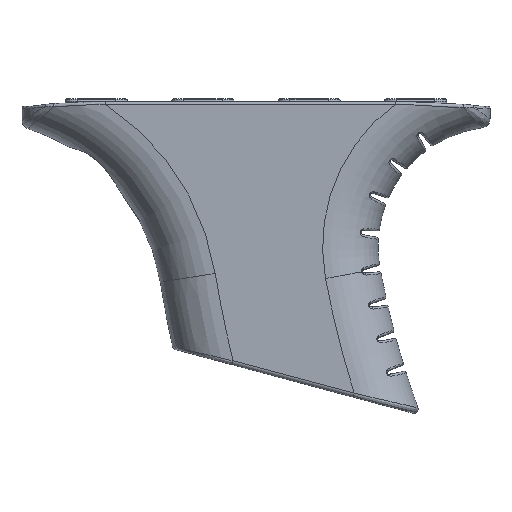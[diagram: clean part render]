
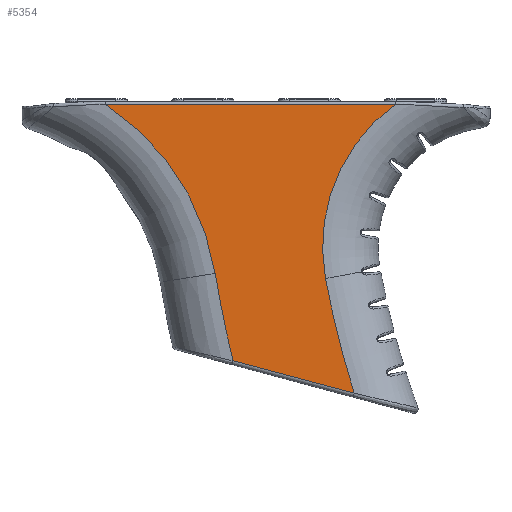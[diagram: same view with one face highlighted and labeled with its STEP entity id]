
A CAD part, left-side view. The second image highlights one B-rep face of the part: STEP entity #5354.
In plain terms, the highlighted planar face has unit normal (-1, 0, 0).
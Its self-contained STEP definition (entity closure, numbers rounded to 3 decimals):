
#47=PLANE('',#5767);
#331=LINE('',#21706,#554);
#336=LINE('',#21870,#559);
#554=VECTOR('',#6568,10.);
#559=VECTOR('',#6621,11.);
#841=FACE_OUTER_BOUND('',#1180,.T.);
#1180=EDGE_LOOP('',(#4352,#4353,#4354,#4355,#4356,#4357));
#1677=CIRCLE('',#5548,33.);
#1707=CIRCLE('',#5583,177.731);
#1833=CIRCLE('',#5761,198.);
#1838=CIRCLE('',#5768,46.75);
#2016=VERTEX_POINT('',#8795);
#2017=VERTEX_POINT('',#8801);
#2103=VERTEX_POINT('',#15218);
#2363=VERTEX_POINT('',#21693);
#2371=VERTEX_POINT('',#21860);
#2373=VERTEX_POINT('',#21869);
#2556=EDGE_CURVE('',#2017,#2016,#1677,.T.);
#2681=EDGE_CURVE('',#2103,#2017,#1707,.T.);
#3042=EDGE_CURVE('',#2103,#2363,#331,.T.);
#3058=EDGE_CURVE('',#2371,#2363,#1833,.T.);
#3063=EDGE_CURVE('',#2373,#2016,#336,.T.);
#3064=EDGE_CURVE('',#2371,#2373,#1838,.T.);
#4352=ORIENTED_EDGE('',*,*,#3042,.F.);
#4353=ORIENTED_EDGE('',*,*,#2681,.T.);
#4354=ORIENTED_EDGE('',*,*,#2556,.T.);
#4355=ORIENTED_EDGE('',*,*,#3063,.F.);
#4356=ORIENTED_EDGE('',*,*,#3064,.F.);
#4357=ORIENTED_EDGE('',*,*,#3058,.T.);
#5354=ADVANCED_FACE('',(#841),#47,.T.);
#5548=AXIS2_PLACEMENT_3D('',#8802,#6082,#6083);
#5583=AXIS2_PLACEMENT_3D('',#15219,#6155,#6156);
#5761=AXIS2_PLACEMENT_3D('',#21861,#6607,#6608);
#5767=AXIS2_PLACEMENT_3D('',#21868,#6619,#6620);
#5768=AXIS2_PLACEMENT_3D('',#21871,#6622,#6623);
#6082=DIRECTION('center_axis',(1.,0.,0.));
#6083=DIRECTION('ref_axis',(0.,0.915,0.402));
#6155=DIRECTION('center_axis',(1.,0.,0.));
#6156=DIRECTION('ref_axis',(0.,0.957,-0.289));
#6568=DIRECTION('',(0.,0.966,0.259));
#6607=DIRECTION('center_axis',(-1.,0.,0.));
#6608=DIRECTION('ref_axis',(0.,0.965,-0.26));
#6619=DIRECTION('center_axis',(-1.,0.,0.));
#6620=DIRECTION('ref_axis',(0.,-1.,0.));
#6621=DIRECTION('',(0.,-1.,0.));
#6622=DIRECTION('center_axis',(-1.,0.,0.));
#6623=DIRECTION('ref_axis',(0.,0.,
-1.));
#8795=CARTESIAN_POINT('',(-11.75,-150.309,103.431));
#8801=CARTESIAN_POINT('',(-11.75,-137.171,70.663));
#8802=CARTESIAN_POINT('Origin',(-11.75,-169.62,76.67));
#15218=CARTESIAN_POINT('',(-11.75,-142.581,49.089));
#15219=CARTESIAN_POINT('Origin',(-11.75,-311.932,103.019));
#21693=CARTESIAN_POINT('',(-11.75,-119.796,55.186));
#21706=CARTESIAN_POINT('',(-11.75,-197.912,34.282));
#21860=CARTESIAN_POINT('',(-11.75,-116.435,71.634));
#21861=CARTESIAN_POINT('Origin',(-11.75,-311.932,103.019));
#21868=CARTESIAN_POINT('Origin',(-11.75,-300.939,103.019));
#21869=CARTESIAN_POINT('',(-11.75,-95.74,103.431));
#21870=CARTESIAN_POINT('',(-11.75,-80.101,103.431));
#21871=CARTESIAN_POINT('Origin',(-11.75,-70.276,64.224));
